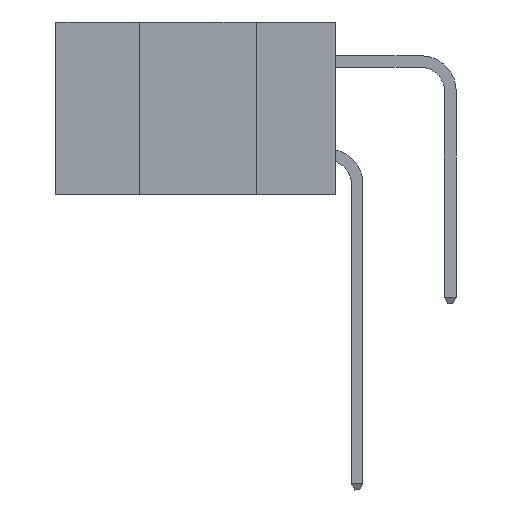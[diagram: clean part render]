
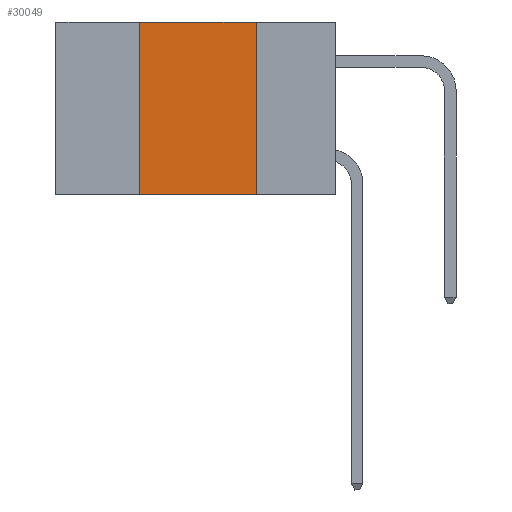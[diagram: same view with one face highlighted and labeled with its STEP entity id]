
A CAD part, left-side view. The second image highlights one B-rep face of the part: STEP entity #30049.
In plain terms, the highlighted planar face has unit normal (-1, 0, 0).
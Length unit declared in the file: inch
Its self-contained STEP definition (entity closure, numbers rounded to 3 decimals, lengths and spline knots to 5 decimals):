
#313 = CARTESIAN_POINT ( 'NONE',  ( 0., 0.17, 0. ) ) ;
#439 = DIRECTION ( 'NONE',  ( 1., 0., 0. ) ) ;
#1108 = DIRECTION ( 'NONE',  ( 0., -1., 0. ) ) ;
#1305 = ORIENTED_EDGE ( 'NONE', *, *, #5567, .T. ) ;
#1626 = EDGE_CURVE ( 'NONE', #3032, #5051, #6177, .T. ) ;
#2080 = VECTOR ( 'NONE', #27274, 39.37008 ) ;
#3032 = VERTEX_POINT ( 'NONE', #7898 ) ;
#3085 = VERTEX_POINT ( 'NONE', #32328 ) ;
#5051 = VERTEX_POINT ( 'NONE', #15683 ) ;
#5567 = EDGE_CURVE ( 'NONE', #25486, #5051, #10035, .T. ) ;
#5710 = CARTESIAN_POINT ( 'NONE',  ( 0., 0.6, -0.37 ) ) ;
#6177 = LINE ( 'NONE', #313, #21758 ) ;
#6569 = AXIS2_PLACEMENT_3D ( 'NONE', #24535, #439, #22076 ) ;
#7171 = EDGE_CURVE ( 'NONE', #3085, #3032, #28040, .T. ) ;
#7898 = CARTESIAN_POINT ( 'NONE',  ( 0., 0.17, 0. ) ) ;
#10035 = LINE ( 'NONE', #5710, #31872 ) ;
#13372 = LINE ( 'NONE', #22010, #2080 ) ;
#13770 = EDGE_CURVE ( 'NONE', #25486, #3085, #13372, .T. ) ;
#13832 = DIRECTION ( 'NONE',  ( 0., -1., 0. ) ) ;
#15683 = CARTESIAN_POINT ( 'NONE',  ( 0., 0.17, -0.37 ) ) ;
#18810 = VECTOR ( 'NONE', #1108, 39.37008 ) ;
#20037 = CARTESIAN_POINT ( 'NONE',  ( 0., 0.6, 0. ) ) ;
#20331 = ORIENTED_EDGE ( 'NONE', *, *, #7171, .F. ) ;
#21109 = CARTESIAN_POINT ( 'NONE',  ( 0., 0.42, -0.37 ) ) ;
#21758 = VECTOR ( 'NONE', #32706, 39.37008 ) ;
#22010 = CARTESIAN_POINT ( 'NONE',  ( 0., 0.42, 0. ) ) ;
#22076 = DIRECTION ( 'NONE',  ( 0., 0., -1. ) ) ;
#24535 = CARTESIAN_POINT ( 'NONE',  ( 0., 0.6, 0. ) ) ;
#24757 = EDGE_LOOP ( 'NONE', ( #27735, #20331, #34750, #1305 ) ) ;
#25486 = VERTEX_POINT ( 'NONE', #21109 ) ;
#26549 = FACE_OUTER_BOUND ( 'NONE', #24757, .T. ) ;
#27274 = DIRECTION ( 'NONE',  ( 0., 0., 1. ) ) ;
#27735 = ORIENTED_EDGE ( 'NONE', *, *, #1626, .F. ) ;
#28040 = LINE ( 'NONE', #20037, #18810 ) ;
#30049 = ADVANCED_FACE ( 'NONE', ( #26549 ), #32491, .F. ) ;
#31872 = VECTOR ( 'NONE', #13832, 39.37008 ) ;
#32328 = CARTESIAN_POINT ( 'NONE',  ( 0., 0.42, 0. ) ) ;
#32491 = PLANE ( 'NONE',  #6569 ) ;
#32706 = DIRECTION ( 'NONE',  ( 0., 0., -1. ) ) ;
#34750 = ORIENTED_EDGE ( 'NONE', *, *, #13770, .F. ) ;
